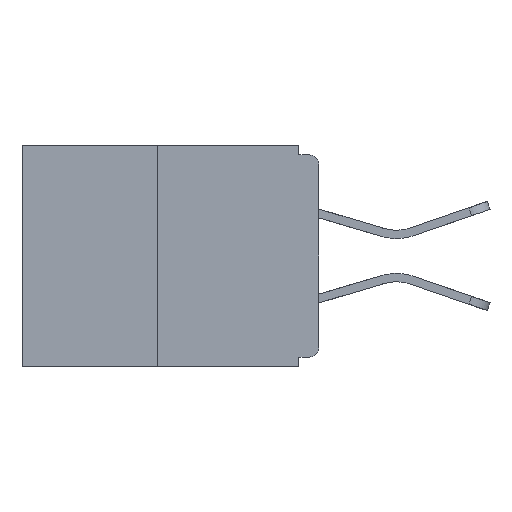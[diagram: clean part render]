
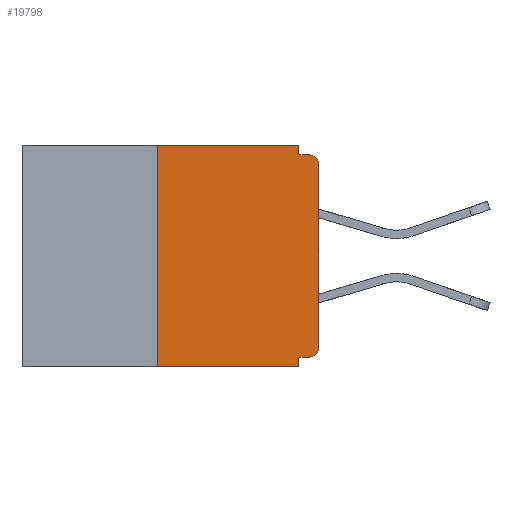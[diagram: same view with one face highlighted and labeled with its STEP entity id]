
A CAD part, left-side view. The second image highlights one B-rep face of the part: STEP entity #19798.
In plain terms, the highlighted planar face has unit normal (-1, 0, 0).
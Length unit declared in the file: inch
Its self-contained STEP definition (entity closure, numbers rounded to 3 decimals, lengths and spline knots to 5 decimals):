
#173 = AXIS2_PLACEMENT_3D ( 'NONE', #12600, #18931, #1649 ) ;
#286 = CARTESIAN_POINT ( 'NONE',  ( 0., 0.46, -0.343 ) ) ;
#587 = LINE ( 'NONE', #6713, #19449 ) ;
#714 = EDGE_CURVE ( 'NONE', #19152, #10830, #7010, .T. ) ;
#1058 = AXIS2_PLACEMENT_3D ( 'NONE', #3028, #1783, #15748 ) ;
#1206 = VERTEX_POINT ( 'NONE', #14053 ) ;
#1307 = DIRECTION ( 'NONE',  ( 0., 0., -1. ) ) ;
#1498 = ORIENTED_EDGE ( 'NONE', *, *, #18269, .T. ) ;
#1548 = LINE ( 'NONE', #4462, #16391 ) ;
#1649 = DIRECTION ( 'NONE',  ( 0., 0., -1. ) ) ;
#1783 = DIRECTION ( 'NONE',  ( -1., 0., 0. ) ) ;
#2127 = ORIENTED_EDGE ( 'NONE', *, *, #4394, .F. ) ;
#2488 = VERTEX_POINT ( 'NONE', #15868 ) ;
#3028 = CARTESIAN_POINT ( 'NONE',  ( 0., 0.015, -0.03 ) ) ;
#3576 = ORIENTED_EDGE ( 'NONE', *, *, #15829, .F. ) ;
#4321 = CARTESIAN_POINT ( 'NONE',  ( 0., 0., -0.328 ) ) ;
#4394 = EDGE_CURVE ( 'NONE', #2488, #1206, #19960, .T. ) ;
#4415 = CARTESIAN_POINT ( 'NONE',  ( 0., 0., -0.03 ) ) ;
#4462 = CARTESIAN_POINT ( 'NONE',  ( 0., 0.031, 0. ) ) ;
#5275 = EDGE_CURVE ( 'NONE', #17085, #19152, #12832, .T. ) ;
#5594 = LINE ( 'NONE', #4321, #14187 ) ;
#6200 = CARTESIAN_POINT ( 'NONE',  ( 0., 0.015, -0.328 ) ) ;
#6394 = CARTESIAN_POINT ( 'NONE',  ( 0., 0.46, 0. ) ) ;
#6647 = EDGE_CURVE ( 'NONE', #15113, #16783, #1548, .T. ) ;
#6713 = CARTESIAN_POINT ( 'NONE',  ( 0., 0., -0.015 ) ) ;
#7010 = LINE ( 'NONE', #18046, #14825 ) ;
#7147 = ORIENTED_EDGE ( 'NONE', *, *, #6647, .F. ) ;
#7150 = VECTOR ( 'NONE', #17138, 39.37008 ) ;
#7204 = VECTOR ( 'NONE', #12997, 39.37008 ) ;
#7488 = EDGE_LOOP ( 'NONE', ( #18726, #3576, #1498, #2127, #11096, #11241, #13077, #14887, #8953, #7147 ) ) ;
#7491 = CARTESIAN_POINT ( 'NONE',  ( 0., 0., -0.313 ) ) ;
#8066 = EDGE_CURVE ( 'NONE', #16783, #11870, #587, .T. ) ;
#8209 = LINE ( 'NONE', #286, #13188 ) ;
#8779 = CARTESIAN_POINT ( 'NONE',  ( 0., 0.25, 0. ) ) ;
#8953 = ORIENTED_EDGE ( 'NONE', *, *, #8066, .F. ) ;
#9125 = CARTESIAN_POINT ( 'NONE',  ( 0., 0.031, 0. ) ) ;
#9424 = FACE_OUTER_BOUND ( 'NONE', #7488, .T. ) ;
#10181 = CARTESIAN_POINT ( 'NONE',  ( 0., 0.46, 0. ) ) ;
#10787 = CARTESIAN_POINT ( 'NONE',  ( 0., 0.031, -0.343 ) ) ;
#10830 = VERTEX_POINT ( 'NONE', #4415 ) ;
#11096 = ORIENTED_EDGE ( 'NONE', *, *, #19667, .F. ) ;
#11241 = ORIENTED_EDGE ( 'NONE', *, *, #5275, .T. ) ;
#11384 = EDGE_CURVE ( 'NONE', #10830, #11870, #20348, .T. ) ;
#11542 = DIRECTION ( 'NONE',  ( 0., -1., 0. ) ) ;
#11870 = VERTEX_POINT ( 'NONE', #12700 ) ;
#11926 = DIRECTION ( 'NONE',  ( 0., 0., 1. ) ) ;
#11942 = DIRECTION ( 'NONE',  ( 0., -1., 0. ) ) ;
#11958 = DIRECTION ( 'NONE',  ( 0., 1., 0. ) ) ;
#12504 = CARTESIAN_POINT ( 'NONE',  ( 0., 0.25, 0. ) ) ;
#12600 = CARTESIAN_POINT ( 'NONE',  ( 0., 0.015, -0.313 ) ) ;
#12602 = VERTEX_POINT ( 'NONE', #17298 ) ;
#12700 = CARTESIAN_POINT ( 'NONE',  ( 0., 0.015, -0.015 ) ) ;
#12832 = CIRCLE ( 'NONE', #173, 0.015 ) ;
#12929 = VERTEX_POINT ( 'NONE', #12504 ) ;
#12997 = DIRECTION ( 'NONE',  ( 0., -1., 0. ) ) ;
#13077 = ORIENTED_EDGE ( 'NONE', *, *, #714, .T. ) ;
#13188 = VECTOR ( 'NONE', #11542, 39.37008 ) ;
#13920 = PLANE ( 'NONE',  #16177 ) ;
#14053 = CARTESIAN_POINT ( 'NONE',  ( 0., 0.031, -0.343 ) ) ;
#14187 = VECTOR ( 'NONE', #11958, 39.37008 ) ;
#14825 = VECTOR ( 'NONE', #11926, 39.37008 ) ;
#14881 = LINE ( 'NONE', #10181, #7204 ) ;
#14887 = ORIENTED_EDGE ( 'NONE', *, *, #11384, .T. ) ;
#15020 = LINE ( 'NONE', #8779, #19732 ) ;
#15113 = VERTEX_POINT ( 'NONE', #9125 ) ;
#15588 = DIRECTION ( 'NONE',  ( 1., 0., 0. ) ) ;
#15748 = DIRECTION ( 'NONE',  ( 0., 0., -1. ) ) ;
#15829 = EDGE_CURVE ( 'NONE', #12602, #12929, #15020, .T. ) ;
#15868 = CARTESIAN_POINT ( 'NONE',  ( 0., 0.031, -0.328 ) ) ;
#16177 = AXIS2_PLACEMENT_3D ( 'NONE', #6394, #15588, #1307 ) ;
#16391 = VECTOR ( 'NONE', #18628, 39.37008 ) ;
#16783 = VERTEX_POINT ( 'NONE', #17981 ) ;
#17085 = VERTEX_POINT ( 'NONE', #6200 ) ;
#17138 = DIRECTION ( 'NONE',  ( 0., 0., -1. ) ) ;
#17298 = CARTESIAN_POINT ( 'NONE',  ( 0., 0.25, -0.343 ) ) ;
#17981 = CARTESIAN_POINT ( 'NONE',  ( 0., 0.031, -0.015 ) ) ;
#18046 = CARTESIAN_POINT ( 'NONE',  ( 0., 0., 0. ) ) ;
#18269 = EDGE_CURVE ( 'NONE', #12602, #1206, #8209, .T. ) ;
#18628 = DIRECTION ( 'NONE',  ( 0., 0., -1. ) ) ;
#18726 = ORIENTED_EDGE ( 'NONE', *, *, #19536, .F. ) ;
#18931 = DIRECTION ( 'NONE',  ( -1., 0., 0. ) ) ;
#19152 = VERTEX_POINT ( 'NONE', #7491 ) ;
#19449 = VECTOR ( 'NONE', #11942, 39.37008 ) ;
#19536 = EDGE_CURVE ( 'NONE', #12929, #15113, #14881, .T. ) ;
#19607 = DIRECTION ( 'NONE',  ( 0., 0., 1. ) ) ;
#19667 = EDGE_CURVE ( 'NONE', #17085, #2488, #5594, .T. ) ;
#19732 = VECTOR ( 'NONE', #19607, 39.37008 ) ;
#19798 = ADVANCED_FACE ( 'NONE', ( #9424 ), #13920, .F. ) ;
#19960 = LINE ( 'NONE', #10787, #7150 ) ;
#20348 = CIRCLE ( 'NONE', #1058, 0.015 ) ;
